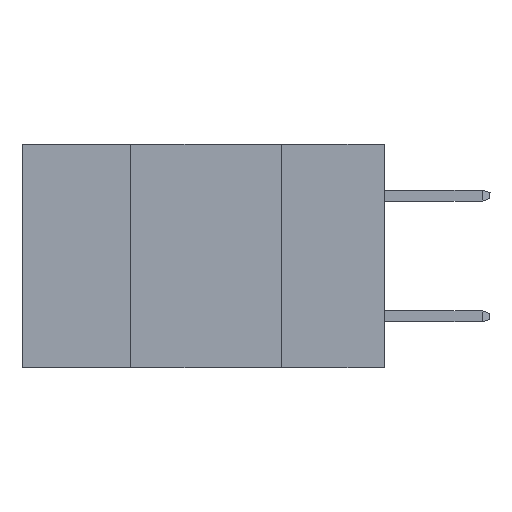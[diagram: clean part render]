
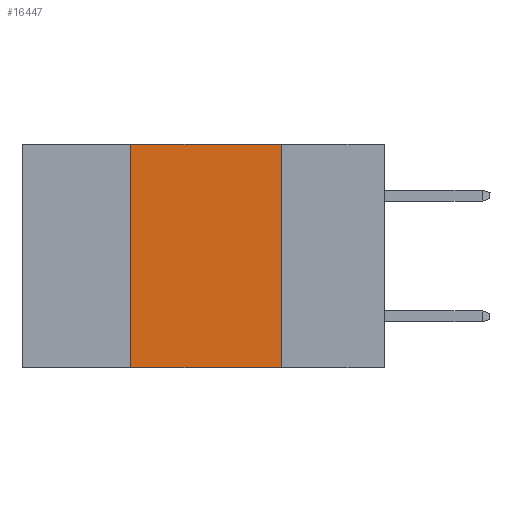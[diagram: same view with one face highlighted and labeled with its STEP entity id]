
A CAD part, left-side view. The second image highlights one B-rep face of the part: STEP entity #16447.
In plain terms, the highlighted planar face has unit normal (-1, 0, 0).
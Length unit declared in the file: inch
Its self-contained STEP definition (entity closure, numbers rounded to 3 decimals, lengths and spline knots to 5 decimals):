
#710 = DIRECTION ( 'NONE',  ( 0., 0., -1. ) ) ;
#1389 = VERTEX_POINT ( 'NONE', #7653 ) ;
#1588 = EDGE_CURVE ( 'NONE', #18835, #1389, #14967, .T. ) ;
#1610 = CARTESIAN_POINT ( 'NONE',  ( 0., 0.42, 0. ) ) ;
#2735 = LINE ( 'NONE', #8728, #4478 ) ;
#4478 = VECTOR ( 'NONE', #8829, 39.37008 ) ;
#5016 = EDGE_LOOP ( 'NONE', ( #10042, #26369, #15079, #12347 ) ) ;
#5376 = CARTESIAN_POINT ( 'NONE',  ( 0., 0.6, 0. ) ) ;
#5456 = VECTOR ( 'NONE', #710, 39.37008 ) ;
#7631 = DIRECTION ( 'NONE',  ( 1., 0., 0. ) ) ;
#7653 = CARTESIAN_POINT ( 'NONE',  ( 0., 0.17, -0.37 ) ) ;
#7957 = AXIS2_PLACEMENT_3D ( 'NONE', #5376, #7631, #21797 ) ;
#8572 = CARTESIAN_POINT ( 'NONE',  ( 0., 0.6, -0.37 ) ) ;
#8728 = CARTESIAN_POINT ( 'NONE',  ( 0., 0.6, 0. ) ) ;
#8829 = DIRECTION ( 'NONE',  ( 0., -1., 0. ) ) ;
#10042 = ORIENTED_EDGE ( 'NONE', *, *, #23603, .F. ) ;
#11720 = LINE ( 'NONE', #28325, #5456 ) ;
#12347 = ORIENTED_EDGE ( 'NONE', *, *, #1588, .T. ) ;
#14967 = LINE ( 'NONE', #8572, #25547 ) ;
#15079 = ORIENTED_EDGE ( 'NONE', *, *, #25039, .F. ) ;
#15652 = LINE ( 'NONE', #1610, #29183 ) ;
#16447 = ADVANCED_FACE ( 'NONE', ( #30100 ), #21696, .F. ) ;
#18567 = CARTESIAN_POINT ( 'NONE',  ( 0., 0.42, -0.37 ) ) ;
#18835 = VERTEX_POINT ( 'NONE', #18567 ) ;
#21696 = PLANE ( 'NONE',  #7957 ) ;
#21797 = DIRECTION ( 'NONE',  ( 0., 0., -1. ) ) ;
#22031 = EDGE_CURVE ( 'NONE', #27036, #29529, #2735, .T. ) ;
#23603 = EDGE_CURVE ( 'NONE', #29529, #1389, #11720, .T. ) ;
#25039 = EDGE_CURVE ( 'NONE', #18835, #27036, #15652, .T. ) ;
#25156 = DIRECTION ( 'NONE',  ( 0., -1., 0. ) ) ;
#25547 = VECTOR ( 'NONE', #25156, 39.37008 ) ;
#26369 = ORIENTED_EDGE ( 'NONE', *, *, #22031, .F. ) ;
#26670 = CARTESIAN_POINT ( 'NONE',  ( 0., 0.17, 0. ) ) ;
#26710 = CARTESIAN_POINT ( 'NONE',  ( 0., 0.42, 0. ) ) ;
#27036 = VERTEX_POINT ( 'NONE', #26710 ) ;
#28325 = CARTESIAN_POINT ( 'NONE',  ( 0., 0.17, 0. ) ) ;
#29183 = VECTOR ( 'NONE', #29670, 39.37008 ) ;
#29529 = VERTEX_POINT ( 'NONE', #26670 ) ;
#29670 = DIRECTION ( 'NONE',  ( 0., 0., 1. ) ) ;
#30100 = FACE_OUTER_BOUND ( 'NONE', #5016, .T. ) ;
